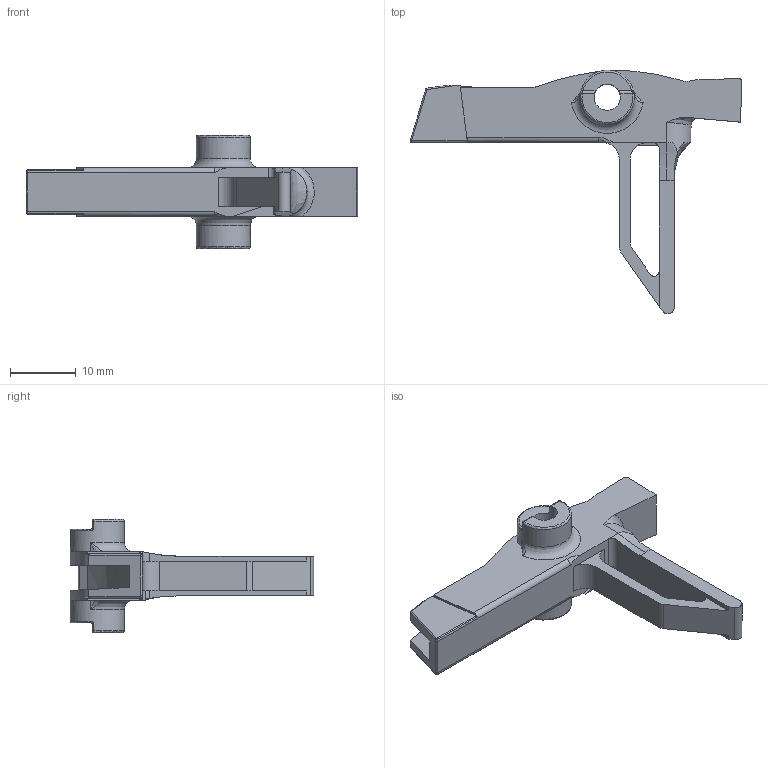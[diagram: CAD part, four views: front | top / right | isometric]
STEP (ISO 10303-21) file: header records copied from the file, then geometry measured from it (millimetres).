
FILE_DESCRIPTION(/* description */ (''),/* implementation_level */ '2;1');
FILE_NAME(/* name */ 'Trigger.step',/* time_stamp */ '2022-05-12T09:42:19-06:00',/* author */ (''),/* organization */ (''),/* preprocessor_version */ 'ST-DEVELOPER v18.1',/* originating_system */ 'Autodesk Translation Framework v10.10.0.1391',/* authorisation */ '');
FILE_SCHEMA (('AUTOMOTIVE_DESIGN { 1 0 10303 214 3 1 1 }'));
Length unit declared in the file: millimetre
Products named in the file (1): Trigger custom
Bounding box: 50.28 x 36.89 x 17.17 mm (x, y, z)
Volume: 3022.9 mm3; surface area: 3250 mm2
Topology: 1 solids, 1 shells, 133 faces, 374 edges, 236 vertices
Faces by surface type: cylinder 51, plane 47, bspline 22, torus 7, sphere 6
Full cylindrical faces by diameter (mm): 3.962 x2, 4.166 x1, 8.179 x2
Entity records: 5752 total; most frequent: CARTESIAN_POINT 2359, ORIENTED_EDGE 742, DIRECTION 674, EDGE_CURVE 371, AXIS2_PLACEMENT_3D 252, VERTEX_POINT 236, LINE 170, VECTOR 170
